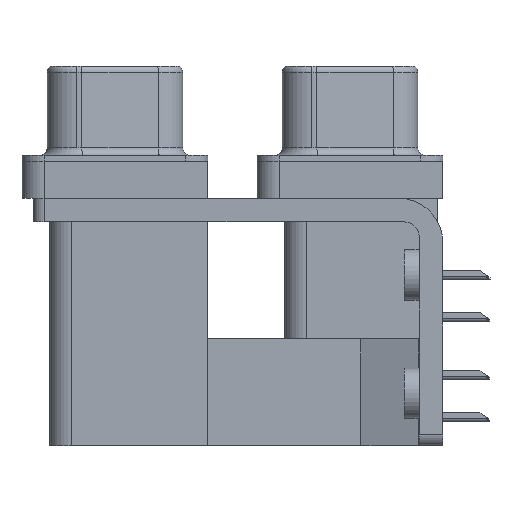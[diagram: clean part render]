
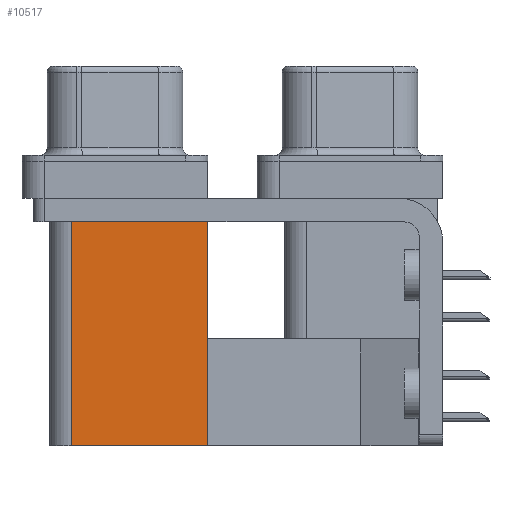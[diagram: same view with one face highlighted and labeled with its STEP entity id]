
A CAD part, left-side view. The second image highlights one B-rep face of the part: STEP entity #10517.
In plain terms, the highlighted planar face has unit normal (-1, 0, 0).
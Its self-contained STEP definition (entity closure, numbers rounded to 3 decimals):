
#167 = DIRECTION ( 'NONE',  ( 0., 0., 1. ) ) ;
#191 = ORIENTED_EDGE ( 'NONE', *, *, #4768, .T. ) ;
#371 = CARTESIAN_POINT ( 'NONE',  ( 3.79, 18.8, -2.5 ) ) ;
#687 = CARTESIAN_POINT ( 'NONE',  ( 3.79, 9.6, -19.2 ) ) ;
#815 = DIRECTION ( 'NONE',  ( 0., 1., 0. ) ) ;
#1105 = CARTESIAN_POINT ( 'NONE',  ( 3.79, 9.6, -2.5 ) ) ;
#1418 = LINE ( 'NONE', #13827, #10247 ) ;
#2196 = ORIENTED_EDGE ( 'NONE', *, *, #25162, .F. ) ;
#2519 = LINE ( 'NONE', #687, #10001 ) ;
#4768 = EDGE_CURVE ( 'NONE', #15994, #14569, #2519, .T. ) ;
#5001 = EDGE_LOOP ( 'NONE', ( #16403, #21491, #2196, #191 ) ) ;
#6424 = LINE ( 'NONE', #12459, #13748 ) ;
#6692 = CARTESIAN_POINT ( 'NONE',  ( 3.79, 18.8, -19.2 ) ) ;
#7594 = CARTESIAN_POINT ( 'NONE',  ( 3.79, 9.6, -19.2 ) ) ;
#9734 = LINE ( 'NONE', #23683, #9776 ) ;
#9776 = VECTOR ( 'NONE', #16004, 1000. ) ;
#10001 = VECTOR ( 'NONE', #167, 1000. ) ;
#10247 = VECTOR ( 'NONE', #19312, 1000. ) ;
#10517 = ADVANCED_FACE ( 'NONE', ( #11010 ), #13243, .F. ) ;
#11010 = FACE_OUTER_BOUND ( 'NONE', #5001, .T. ) ;
#12459 = CARTESIAN_POINT ( 'NONE',  ( 3.79, 9.6, -2.5 ) ) ;
#13243 = PLANE ( 'NONE',  #23541 ) ;
#13748 = VECTOR ( 'NONE', #815, 1000. ) ;
#13827 = CARTESIAN_POINT ( 'NONE',  ( 3.79, 9.6, -19.2 ) ) ;
#14569 = VERTEX_POINT ( 'NONE', #1105 ) ;
#15016 = VERTEX_POINT ( 'NONE', #6692 ) ;
#15994 = VERTEX_POINT ( 'NONE', #7594 ) ;
#16004 = DIRECTION ( 'NONE',  ( 0., 0., 1. ) ) ;
#16403 = ORIENTED_EDGE ( 'NONE', *, *, #21204, .T. ) ;
#17855 = VERTEX_POINT ( 'NONE', #371 ) ;
#18970 = DIRECTION ( 'NONE',  ( 0., 0., -1. ) ) ;
#19312 = DIRECTION ( 'NONE',  ( 0., 1., 0. ) ) ;
#20790 = CARTESIAN_POINT ( 'NONE',  ( 3.79, 9.6, -19.2 ) ) ;
#21204 = EDGE_CURVE ( 'NONE', #14569, #17855, #6424, .T. ) ;
#21491 = ORIENTED_EDGE ( 'NONE', *, *, #23883, .F. ) ;
#23541 = AXIS2_PLACEMENT_3D ( 'NONE', #20790, #24687, #18970 ) ;
#23683 = CARTESIAN_POINT ( 'NONE',  ( 3.79, 18.8, -19.2 ) ) ;
#23883 = EDGE_CURVE ( 'NONE', #15016, #17855, #9734, .T. ) ;
#24687 = DIRECTION ( 'NONE',  ( 1., 0., 0. ) ) ;
#25162 = EDGE_CURVE ( 'NONE', #15994, #15016, #1418, .T. ) ;
